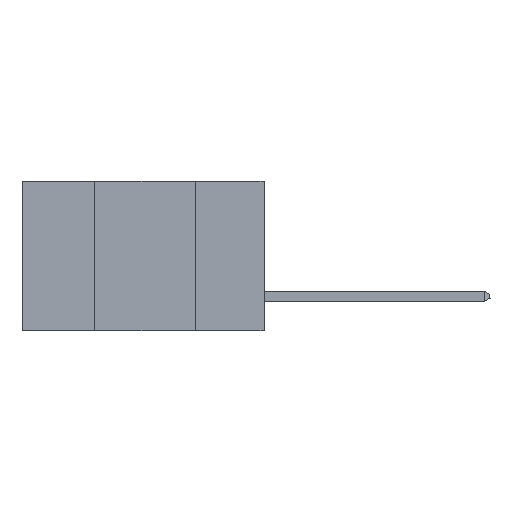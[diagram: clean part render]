
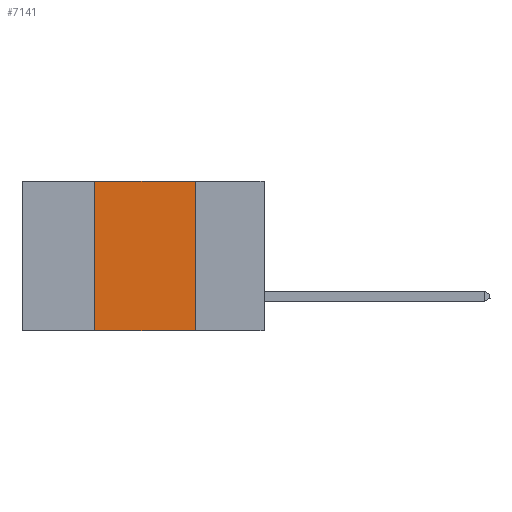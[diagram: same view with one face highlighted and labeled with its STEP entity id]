
A CAD part, left-side view. The second image highlights one B-rep face of the part: STEP entity #7141.
In plain terms, the highlighted planar face has unit normal (-1, 0, 0).
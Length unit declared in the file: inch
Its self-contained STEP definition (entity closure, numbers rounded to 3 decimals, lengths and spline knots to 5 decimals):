
#198 = ORIENTED_EDGE ( 'NONE', *, *, #1613, .T. ) ;
#968 = VERTEX_POINT ( 'NONE', #9284 ) ;
#1511 = DIRECTION ( 'NONE',  ( 0., 0., -1. ) ) ;
#1542 = VECTOR ( 'NONE', #1511, 39.37008 ) ;
#1613 = EDGE_CURVE ( 'NONE', #7277, #11617, #3222, .T. ) ;
#2893 = DIRECTION ( 'NONE',  ( 1., 0., 0. ) ) ;
#2981 = LINE ( 'NONE', #10441, #1542 ) ;
#3012 = CARTESIAN_POINT ( 'NONE',  ( 0., 0.17, -0.37 ) ) ;
#3169 = EDGE_LOOP ( 'NONE', ( #5122, #9736, #13681, #198 ) ) ;
#3222 = LINE ( 'NONE', #7494, #9437 ) ;
#3864 = EDGE_CURVE ( 'NONE', #7277, #968, #11058, .T. ) ;
#3941 = EDGE_CURVE ( 'NONE', #968, #12965, #7895, .T. ) ;
#5122 = ORIENTED_EDGE ( 'NONE', *, *, #6603, .F. ) ;
#5124 = DIRECTION ( 'NONE',  ( 0., 0., -1. ) ) ;
#6204 = PLANE ( 'NONE',  #14108 ) ;
#6259 = CARTESIAN_POINT ( 'NONE',  ( 0., 0.17, 0. ) ) ;
#6603 = EDGE_CURVE ( 'NONE', #12965, #11617, #2981, .T. ) ;
#7141 = ADVANCED_FACE ( 'NONE', ( #8295 ), #6204, .F. ) ;
#7277 = VERTEX_POINT ( 'NONE', #14519 ) ;
#7414 = CARTESIAN_POINT ( 'NONE',  ( 0., 0.6, 0. ) ) ;
#7494 = CARTESIAN_POINT ( 'NONE',  ( 0., 0.6, -0.37 ) ) ;
#7833 = CARTESIAN_POINT ( 'NONE',  ( 0., 0.42, 0. ) ) ;
#7895 = LINE ( 'NONE', #10582, #8759 ) ;
#8295 = FACE_OUTER_BOUND ( 'NONE', #3169, .T. ) ;
#8759 = VECTOR ( 'NONE', #10486, 39.37008 ) ;
#9284 = CARTESIAN_POINT ( 'NONE',  ( 0., 0.42, 0. ) ) ;
#9437 = VECTOR ( 'NONE', #13082, 39.37008 ) ;
#9736 = ORIENTED_EDGE ( 'NONE', *, *, #3941, .F. ) ;
#10074 = DIRECTION ( 'NONE',  ( 0., 0., 1. ) ) ;
#10441 = CARTESIAN_POINT ( 'NONE',  ( 0., 0.17, 0. ) ) ;
#10486 = DIRECTION ( 'NONE',  ( 0., -1., 0. ) ) ;
#10582 = CARTESIAN_POINT ( 'NONE',  ( 0., 0.6, 0. ) ) ;
#11058 = LINE ( 'NONE', #7833, #13744 ) ;
#11617 = VERTEX_POINT ( 'NONE', #3012 ) ;
#12965 = VERTEX_POINT ( 'NONE', #6259 ) ;
#13082 = DIRECTION ( 'NONE',  ( 0., -1., 0. ) ) ;
#13681 = ORIENTED_EDGE ( 'NONE', *, *, #3864, .F. ) ;
#13744 = VECTOR ( 'NONE', #10074, 39.37008 ) ;
#14108 = AXIS2_PLACEMENT_3D ( 'NONE', #7414, #2893, #5124 ) ;
#14519 = CARTESIAN_POINT ( 'NONE',  ( 0., 0.42, -0.37 ) ) ;
